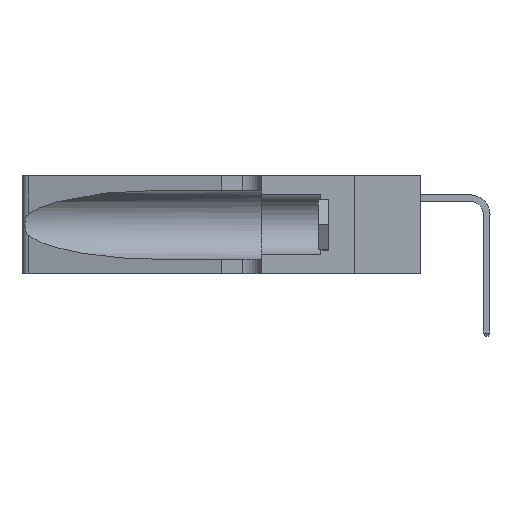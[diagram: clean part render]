
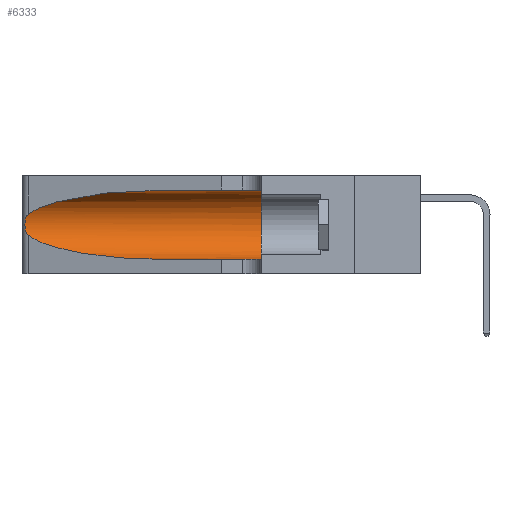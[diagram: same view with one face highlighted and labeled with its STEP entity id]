
A CAD part, left-side view. The second image highlights one B-rep face of the part: STEP entity #6333.
In plain terms, the highlighted cylindrical face has radius 3.308 mm (diameter 6.617 mm), a partial arc.
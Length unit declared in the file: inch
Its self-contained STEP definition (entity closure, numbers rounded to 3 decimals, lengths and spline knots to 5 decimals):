
#125 = VERTEX_POINT ( 'NONE', #6117 ) ;
#459 = CARTESIAN_POINT ( 'NONE',  ( 0.1305, 1.61858, 0.185 ) ) ;
#1026 = ORIENTED_EDGE ( 'NONE', *, *, #22821, .F. ) ;
#1574 = CARTESIAN_POINT ( 'NONE',  ( 0.25854, 1.2359, 0.20912 ) ) ;
#2133 = CARTESIAN_POINT ( 'NONE',  ( 0.25487, 1.22718, 0.22369 ) ) ;
#2591 = DIRECTION ( 'NONE',  ( 0., 0., -1. ) ) ;
#2810 =( BOUNDED_CURVE ( )  B_SPLINE_CURVE ( 3, ( #19658, #7612, #9658, #23756 ),
 .UNSPECIFIED., .F., .F. ) 
 B_SPLINE_CURVE_WITH_KNOTS ( ( 4, 4 ),
 ( 3.44316, 4.71239 ),
 .UNSPECIFIED. ) 
 CURVE ( )  GEOMETRIC_REPRESENTATION_ITEM ( )  RATIONAL_B_SPLINE_CURVE ( ( 1., 0.87, 0.87, 1. ) ) 
 REPRESENTATION_ITEM ( '' )  );
#2883 = VECTOR ( 'NONE', #24617, 39.37008 ) ;
#3555 = LINE ( 'NONE', #22606, #2883 ) ;
#3678 = CARTESIAN_POINT ( 'NONE',  ( 0.26075, 1.23896, 0.19203 ) ) ;
#4123 = VERTEX_POINT ( 'NONE', #15848 ) ;
#4539 = AXIS2_PLACEMENT_3D ( 'NONE', #459, #12813, #2591 ) ;
#4889 = ORIENTED_EDGE ( 'NONE', *, *, #19613, .T. ) ;
#5489 = VERTEX_POINT ( 'NONE', #7921 ) ;
#5709 = CARTESIAN_POINT ( 'NONE',  ( 0.25555, 1.22994, 0.2215 ) ) ;
#5788 = CARTESIAN_POINT ( 'NONE',  ( 0.1305, 0.72297, 0.31525 ) ) ;
#5798 = CARTESIAN_POINT ( 'NONE',  ( 0.26017, 1.23833, 0.17102 ) ) ;
#5957 = CARTESIAN_POINT ( 'NONE',  ( 0.1305, 1.61858, 0.05475 ) ) ;
#5958 = CYLINDRICAL_SURFACE ( 'NONE', #4539, 0.13025 ) ;
#6085 = CARTESIAN_POINT ( 'NONE',  ( 0.25487, 1.22718, 0.14631 ) ) ;
#6117 = CARTESIAN_POINT ( 'NONE',  ( 0.1305, 0.35, 0.31525 ) ) ;
#6333 = ADVANCED_FACE ( 'NONE', ( #22112 ), #5958, .F. ) ;
#7612 = CARTESIAN_POINT ( 'NONE',  ( 0.2373, 1.15595, 0.08982 ) ) ;
#7894 = CARTESIAN_POINT ( 'NONE',  ( 0.25789, 1.23486, 0.15765 ) ) ;
#7921 = CARTESIAN_POINT ( 'NONE',  ( 0.1305, 0.72297, 0.05475 ) ) ;
#7933 = EDGE_LOOP ( 'NONE', ( #12402, #9490, #19394, #4889, #1026, #25577 ) ) ;
#9079 = AXIS2_PLACEMENT_3D ( 'NONE', #22271, #10199, #24293 ) ;
#9484 = LINE ( 'NONE', #5957, #24916 ) ;
#9490 = ORIENTED_EDGE ( 'NONE', *, *, #15852, .T. ) ;
#9658 = CARTESIAN_POINT ( 'NONE',  ( 0.18966, 0.96281, 0.05475 ) ) ;
#9825 = EDGE_CURVE ( 'NONE', #22107, #18461, #18943, .T. ) ;
#9884 = CARTESIAN_POINT ( 'NONE',  ( 0.1305, 0.72297, 0.31525 ) ) ;
#9933 = CARTESIAN_POINT ( 'NONE',  ( 0.25555, 1.22993, 0.14849 ) ) ;
#10199 = DIRECTION ( 'NONE',  ( 0., 1., 0. ) ) ;
#10588 = CIRCLE ( 'NONE', #9079, 0.13025 ) ;
#11829 = CARTESIAN_POINT ( 'NONE',  ( 0.18966, 0.96281, 0.31525 ) ) ;
#12402 = ORIENTED_EDGE ( 'NONE', *, *, #9825, .T. ) ;
#12813 = DIRECTION ( 'NONE',  ( 0., -1., 0. ) ) ;
#13834 = CARTESIAN_POINT ( 'NONE',  ( 0.2373, 1.15595, 0.28018 ) ) ;
#13841 = CARTESIAN_POINT ( 'NONE',  ( 0.25787, 1.23484, 0.2124 ) ) ;
#15842 = CARTESIAN_POINT ( 'NONE',  ( 0.26018, 1.23835, 0.19895 ) ) ;
#15848 = CARTESIAN_POINT ( 'NONE',  ( 0.1305, 0.35, 0.05475 ) ) ;
#15852 = EDGE_CURVE ( 'NONE', #18461, #17697, #26440, .T. ) ;
#17697 = VERTEX_POINT ( 'NONE', #6085 ) ;
#17854 = CARTESIAN_POINT ( 'NONE',  ( 0.26075, 1.23896, 0.178 ) ) ;
#18461 = VERTEX_POINT ( 'NONE', #2133 ) ;
#18943 =( BOUNDED_CURVE ( )  B_SPLINE_CURVE ( 3, ( #5788, #11829, #13834, #19916 ),
 .UNSPECIFIED., .F., .F. ) 
 B_SPLINE_CURVE_WITH_KNOTS ( ( 4, 4 ),
 ( 1.5708, 2.84003 ),
 .UNSPECIFIED. ) 
 CURVE ( )  GEOMETRIC_REPRESENTATION_ITEM ( )  RATIONAL_B_SPLINE_CURVE ( ( 1., 0.87, 0.87, 1. ) ) 
 REPRESENTATION_ITEM ( '' )  );
#19394 = ORIENTED_EDGE ( 'NONE', *, *, #25789, .T. ) ;
#19613 = EDGE_CURVE ( 'NONE', #5489, #4123, #9484, .T. ) ;
#19658 = CARTESIAN_POINT ( 'NONE',  ( 0.25487, 1.22718, 0.14631 ) ) ;
#19916 = CARTESIAN_POINT ( 'NONE',  ( 0.25487, 1.22718, 0.22369 ) ) ;
#19926 = CARTESIAN_POINT ( 'NONE',  ( 0.25856, 1.23593, 0.16098 ) ) ;
#21140 = EDGE_CURVE ( 'NONE', #22107, #125, #3555, .T. ) ;
#21908 = CARTESIAN_POINT ( 'NONE',  ( 0.25487, 1.22718, 0.22369 ) ) ;
#22000 = CARTESIAN_POINT ( 'NONE',  ( 0.25639, 1.23186, 0.15144 ) ) ;
#22107 = VERTEX_POINT ( 'NONE', #9884 ) ;
#22112 = FACE_OUTER_BOUND ( 'NONE', #7933, .T. ) ;
#22148 = DIRECTION ( 'NONE',  ( 0., -1., 0. ) ) ;
#22271 = CARTESIAN_POINT ( 'NONE',  ( 0.1305, 0.35, 0.185 ) ) ;
#22606 = CARTESIAN_POINT ( 'NONE',  ( 0.1305, 1.61858, 0.31525 ) ) ;
#22821 = EDGE_CURVE ( 'NONE', #125, #4123, #10588, .T. ) ;
#23756 = CARTESIAN_POINT ( 'NONE',  ( 0.1305, 0.72297, 0.05475 ) ) ;
#24022 = CARTESIAN_POINT ( 'NONE',  ( 0.25487, 1.22718, 0.14631 ) ) ;
#24293 = DIRECTION ( 'NONE',  ( 0., 0., 1. ) ) ;
#24617 = DIRECTION ( 'NONE',  ( 0., -1., 0. ) ) ;
#24916 = VECTOR ( 'NONE', #22148, 39.37008 ) ;
#25577 = ORIENTED_EDGE ( 'NONE', *, *, #21140, .F. ) ;
#25789 = EDGE_CURVE ( 'NONE', #17697, #5489, #2810, .T. ) ;
#25946 = CARTESIAN_POINT ( 'NONE',  ( 0.25639, 1.23184, 0.21858 ) ) ;
#26440 = B_SPLINE_CURVE_WITH_KNOTS ( 'NONE', 3,
 ( #21908, #5709, #25946, #13841, #1574, #15842, #3678, #17854, #5798, #19926, #7894, #22000, #9933, #24022 ),
 .UNSPECIFIED., .F., .F.,
 ( 4, 2, 2, 2, 2, 2, 4 ),
 ( 0., 0.00027, 0.00053, 0.00107, 0.0016, 0.00187, 0.00214 ),
 .UNSPECIFIED. ) ;
